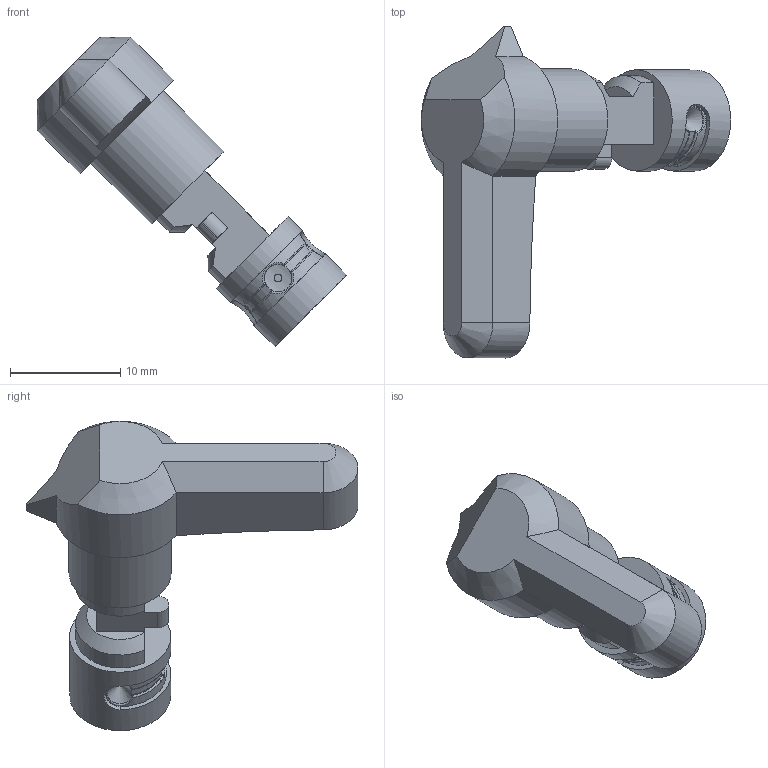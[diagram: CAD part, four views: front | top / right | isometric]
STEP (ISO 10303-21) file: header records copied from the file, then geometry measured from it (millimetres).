
FILE_DESCRIPTION(/* description */ (''),/* implementation_level */ '2;1');
FILE_NAME(/* name */ 'ChoosyBoogleSelectorImproved.stp',/* time_stamp */ '2022-11-09T21:44:13-05:00',/* author */ ('authot'),/* organization */ (''),/* preprocessor_version */ 'ST-DEVELOPER v18.1',/* originating_system */ 'Autodesk Inventor 2022',/* authorisation */ '');
FILE_SCHEMA (('AUTOMOTIVE_DESIGN { 1 0 10303 214 3 1 1 }'));
Length unit declared in the file: inch
Products named in the file (1): YBS2 SS
Bounding box: 28.07 x 30.13 x 28.07 mm (x, y, z)
Volume: 2595.2 mm3; surface area: 1560.6 mm2
Topology: 1 solids, 1 shells, 82 faces, 222 edges, 159 vertices
Faces by surface type: plane 36, bspline 18, cylinder 15, cone 9, torus 4
Full cylindrical faces by diameter (mm): 2.5 x1, 9.2 x1, 9.3 x1
Entity records: 3548 total; most frequent: CARTESIAN_POINT 1584, ORIENTED_EDGE 428, DIRECTION 355, EDGE_CURVE 214, AXIS2_PLACEMENT_3D 140, VERTEX_POINT 138, EDGE_LOOP 86, FACE_OUTER_BOUND 82
